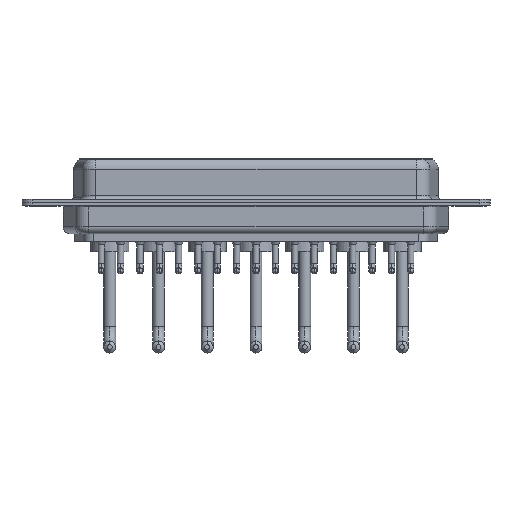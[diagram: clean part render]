
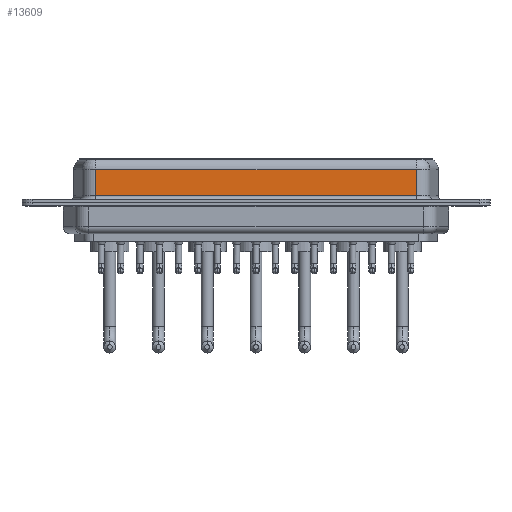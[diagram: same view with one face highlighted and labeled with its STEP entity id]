
A CAD part, front view. The second image highlights one B-rep face of the part: STEP entity #13609.
In plain terms, the highlighted planar face has unit normal (0, -1, 0).
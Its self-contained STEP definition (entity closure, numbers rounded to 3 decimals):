
#95 = CARTESIAN_POINT ( 'NONE',  ( 53.41, -5.375, 0.9 ) ) ;
#1878 = VECTOR ( 'NONE', #9888, 1000. ) ;
#2158 = CARTESIAN_POINT ( 'NONE',  ( 53.41, -5.375, 4.65 ) ) ;
#2232 = EDGE_CURVE ( 'NONE', #3914, #12934, #12554, .T. ) ;
#2700 = CARTESIAN_POINT ( 'NONE',  ( 53.41, -5.375, 6.4 ) ) ;
#2775 = CARTESIAN_POINT ( 'NONE',  ( 7.59, -5.375, 0.9 ) ) ;
#3334 = AXIS2_PLACEMENT_3D ( 'NONE', #4272, #14233, #4176 ) ;
#3414 = VECTOR ( 'NONE', #15267, 1000. ) ;
#3914 = VERTEX_POINT ( 'NONE', #17057 ) ;
#4176 = DIRECTION ( 'NONE',  ( 0., 0., 1. ) ) ;
#4272 = CARTESIAN_POINT ( 'NONE',  ( 53.41, -5.375, 6.4 ) ) ;
#4434 = EDGE_CURVE ( 'NONE', #13091, #12970, #13036, .T. ) ;
#6782 = ORIENTED_EDGE ( 'NONE', *, *, #2232, .T. ) ;
#8436 = ORIENTED_EDGE ( 'NONE', *, *, #11820, .T. ) ;
#9329 = LINE ( 'NONE', #2158, #9584 ) ;
#9490 = CARTESIAN_POINT ( 'NONE',  ( 7.59, -5.375, 6.4 ) ) ;
#9584 = VECTOR ( 'NONE', #9636, 1000. ) ;
#9618 = ORIENTED_EDGE ( 'NONE', *, *, #17354, .T. ) ;
#9636 = DIRECTION ( 'NONE',  ( -1., 0., 0. ) ) ;
#9888 = DIRECTION ( 'NONE',  ( 0., 0., -1. ) ) ;
#11820 = EDGE_CURVE ( 'NONE', #12934, #12970, #16857, .T. ) ;
#12056 = VECTOR ( 'NONE', #18326, 1000. ) ;
#12554 = LINE ( 'NONE', #9490, #3414 ) ;
#12768 = CARTESIAN_POINT ( 'NONE',  ( 53.41, -5.375, 0.9 ) ) ;
#12934 = VERTEX_POINT ( 'NONE', #2775 ) ;
#12970 = VERTEX_POINT ( 'NONE', #95 ) ;
#13036 = LINE ( 'NONE', #2700, #1878 ) ;
#13091 = VERTEX_POINT ( 'NONE', #13871 ) ;
#13609 = ADVANCED_FACE ( 'NONE', ( #18727 ), #14686, .F. ) ;
#13871 = CARTESIAN_POINT ( 'NONE',  ( 53.41, -5.375, 4.65 ) ) ;
#14233 = DIRECTION ( 'NONE',  ( 0., 1., 0. ) ) ;
#14686 = PLANE ( 'NONE',  #3334 ) ;
#15267 = DIRECTION ( 'NONE',  ( 0., 0., -1. ) ) ;
#16504 = EDGE_LOOP ( 'NONE', ( #17997, #9618, #6782, #8436 ) ) ;
#16857 = LINE ( 'NONE', #12768, #12056 ) ;
#17057 = CARTESIAN_POINT ( 'NONE',  ( 7.59, -5.375, 4.65 ) ) ;
#17354 = EDGE_CURVE ( 'NONE', #13091, #3914, #9329, .T. ) ;
#17997 = ORIENTED_EDGE ( 'NONE', *, *, #4434, .F. ) ;
#18326 = DIRECTION ( 'NONE',  ( 1., 0., 0. ) ) ;
#18727 = FACE_OUTER_BOUND ( 'NONE', #16504, .T. ) ;
